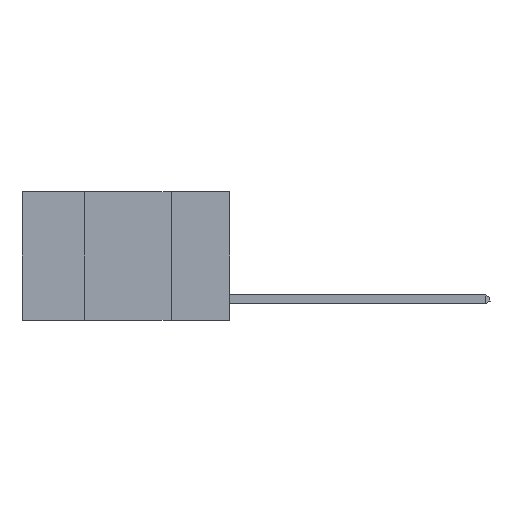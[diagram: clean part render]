
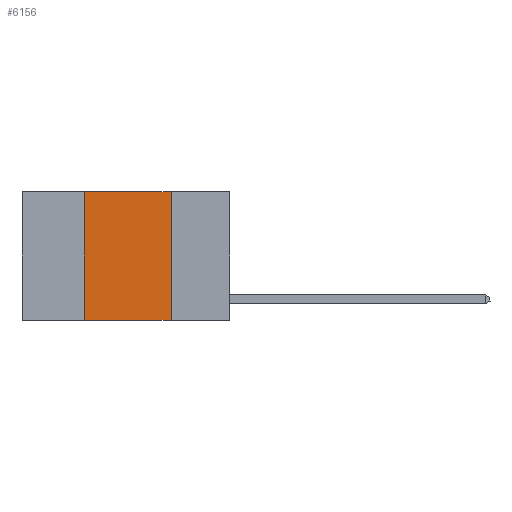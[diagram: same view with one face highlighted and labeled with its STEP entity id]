
A CAD part, left-side view. The second image highlights one B-rep face of the part: STEP entity #6156.
In plain terms, the highlighted planar face has unit normal (-1, 0, 0).
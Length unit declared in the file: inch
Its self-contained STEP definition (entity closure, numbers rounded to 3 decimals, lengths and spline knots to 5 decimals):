
#77 = DIRECTION ( 'NONE',  ( 1., 0., 0. ) ) ;
#242 = ORIENTED_EDGE ( 'NONE', *, *, #11146, .F. ) ;
#285 = ORIENTED_EDGE ( 'NONE', *, *, #3917, .F. ) ;
#368 = CARTESIAN_POINT ( 'NONE',  ( 0., 0.42, 0. ) ) ;
#463 = VERTEX_POINT ( 'NONE', #8525 ) ;
#980 = EDGE_LOOP ( 'NONE', ( #242, #285, #13680, #2066 ) ) ;
#1754 = VERTEX_POINT ( 'NONE', #3410 ) ;
#1868 = LINE ( 'NONE', #10434, #4394 ) ;
#2045 = LINE ( 'NONE', #368, #10579 ) ;
#2066 = ORIENTED_EDGE ( 'NONE', *, *, #9501, .T. ) ;
#2895 = CARTESIAN_POINT ( 'NONE',  ( 0., 0.6, 0. ) ) ;
#3251 = LINE ( 'NONE', #11800, #11744 ) ;
#3410 = CARTESIAN_POINT ( 'NONE',  ( 0., 0.42, -0.37 ) ) ;
#3917 = EDGE_CURVE ( 'NONE', #463, #11327, #6754, .T. ) ;
#4323 = CARTESIAN_POINT ( 'NONE',  ( 0., 0.17, 0. ) ) ;
#4394 = VECTOR ( 'NONE', #8259, 39.37008 ) ;
#6156 = ADVANCED_FACE ( 'NONE', ( #9176 ), #9688, .F. ) ;
#6513 = CARTESIAN_POINT ( 'NONE',  ( 0., 0.6, 0. ) ) ;
#6754 = LINE ( 'NONE', #2895, #12712 ) ;
#6814 = DIRECTION ( 'NONE',  ( 0., 0., 1. ) ) ;
#7330 = VERTEX_POINT ( 'NONE', #12617 ) ;
#7584 = DIRECTION ( 'NONE',  ( 0., 0., -1. ) ) ;
#8259 = DIRECTION ( 'NONE',  ( 0., 0., -1. ) ) ;
#8525 = CARTESIAN_POINT ( 'NONE',  ( 0., 0.42, 0. ) ) ;
#9176 = FACE_OUTER_BOUND ( 'NONE', #980, .T. ) ;
#9501 = EDGE_CURVE ( 'NONE', #1754, #7330, #3251, .T. ) ;
#9620 = DIRECTION ( 'NONE',  ( 0., -1., 0. ) ) ;
#9688 = PLANE ( 'NONE',  #12404 ) ;
#10244 = EDGE_CURVE ( 'NONE', #1754, #463, #2045, .T. ) ;
#10434 = CARTESIAN_POINT ( 'NONE',  ( 0., 0.17, 0. ) ) ;
#10579 = VECTOR ( 'NONE', #6814, 39.37008 ) ;
#11146 = EDGE_CURVE ( 'NONE', #11327, #7330, #1868, .T. ) ;
#11327 = VERTEX_POINT ( 'NONE', #4323 ) ;
#11421 = DIRECTION ( 'NONE',  ( 0., -1., 0. ) ) ;
#11744 = VECTOR ( 'NONE', #9620, 39.37008 ) ;
#11800 = CARTESIAN_POINT ( 'NONE',  ( 0., 0.6, -0.37 ) ) ;
#12404 = AXIS2_PLACEMENT_3D ( 'NONE', #6513, #77, #7584 ) ;
#12617 = CARTESIAN_POINT ( 'NONE',  ( 0., 0.17, -0.37 ) ) ;
#12712 = VECTOR ( 'NONE', #11421, 39.37008 ) ;
#13680 = ORIENTED_EDGE ( 'NONE', *, *, #10244, .F. ) ;
